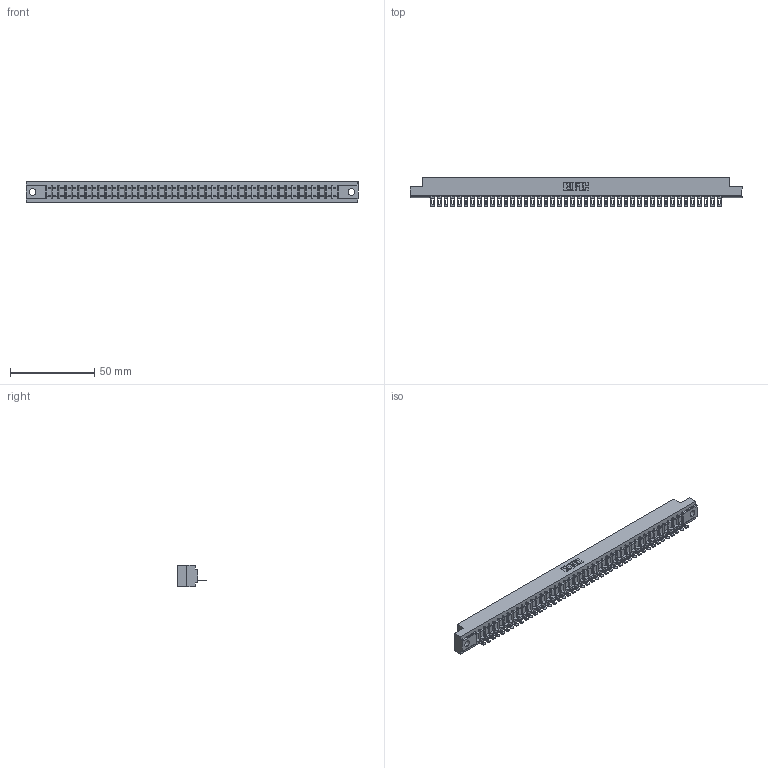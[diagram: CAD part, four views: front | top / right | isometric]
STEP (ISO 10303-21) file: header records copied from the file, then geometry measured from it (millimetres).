
FILE_DESCRIPTION (( 'STEP AP203' ), '1' );
FILE_NAME ('357-044-501-104.STEP', '2019-09-17T11:28:10', ( '' ), ( '' ), 'SwSTEP 2.0', 'SolidWorks 2016', '' );
FILE_SCHEMA (( 'CONFIG_CONTROL_DESIGN' ));
Length unit declared in the file: inch
Products named in the file (3): 357-044-501-104; 307 Part_.156 Dia Mounting Holes; 307-290-002_501
Assembly tree (45 placements, depth 2):
  357-044-501-104
    307 Part_.156 Dia Mounting Holes
    307-290-002_501  x44
Bounding box: 197.36 x 17.42 x 12.7 mm (x, y, z)
Volume: 21067.1 mm3; surface area: 26665.6 mm2
Topology: 45 solids, 45 shells, 3521 faces, 10831 edges, 7098 vertices
Faces by surface type: plane 2020, cylinder 1411, sphere 90
Entity records: 38686 total; most frequent: CARTESIAN_POINT 6530, ORIENTED_EDGE 6518, DIRECTION 6339, EDGE_CURVE 3259, LINE 2501, VECTOR 2501, VERTEX_POINT 2110, AXIS2_PLACEMENT_3D 1919
